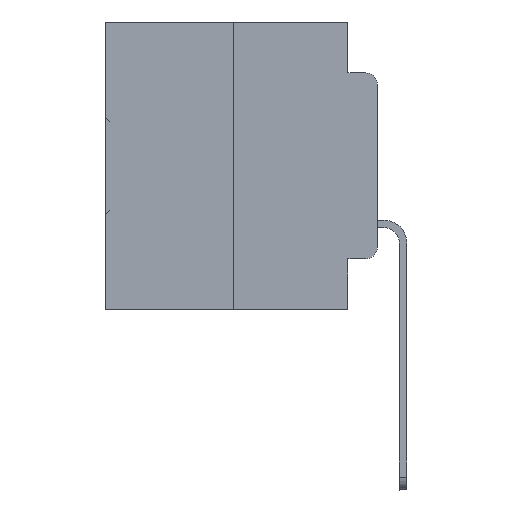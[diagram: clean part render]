
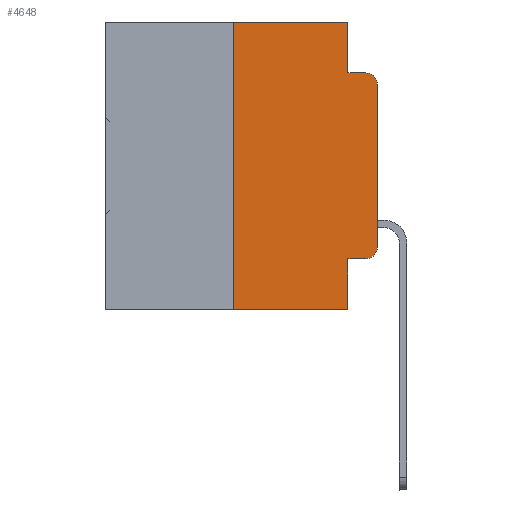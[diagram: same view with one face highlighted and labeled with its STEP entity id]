
A CAD part, left-side view. The second image highlights one B-rep face of the part: STEP entity #4648.
In plain terms, the highlighted planar face has unit normal (-1, 0, 0).
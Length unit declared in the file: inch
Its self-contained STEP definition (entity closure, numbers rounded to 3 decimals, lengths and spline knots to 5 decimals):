
#615 = DIRECTION ( 'NONE',  ( 0., 0., 1. ) ) ;
#1331 = CARTESIAN_POINT ( 'NONE',  ( 0., 0.051, 0. ) ) ;
#1469 = ORIENTED_EDGE ( 'NONE', *, *, #10704, .T. ) ;
#1869 = VECTOR ( 'NONE', #31342, 39.37008 ) ;
#2814 = DIRECTION ( 'NONE',  ( 0., -1., 0. ) ) ;
#2826 = LINE ( 'NONE', #29893, #21544 ) ;
#3425 = EDGE_CURVE ( 'NONE', #15774, #3738, #33092, .T. ) ;
#3437 = CARTESIAN_POINT ( 'NONE',  ( 0., 0.051, 0. ) ) ;
#3597 = VECTOR ( 'NONE', #5594, 39.37008 ) ;
#3738 = VERTEX_POINT ( 'NONE', #4892 ) ;
#3865 = DIRECTION ( 'NONE',  ( 0., 0., -1. ) ) ;
#4002 = DIRECTION ( 'NONE',  ( 0., -1., 0. ) ) ;
#4027 = CARTESIAN_POINT ( 'NONE',  ( 0., 0., -0.3915 ) ) ;
#4268 = ORIENTED_EDGE ( 'NONE', *, *, #32082, .T. ) ;
#4648 = ADVANCED_FACE ( 'NONE', ( #30995 ), #21522, .F. ) ;
#4735 = VECTOR ( 'NONE', #23062, 39.37008 ) ;
#4868 = LINE ( 'NONE', #16063, #3597 ) ;
#4892 = CARTESIAN_POINT ( 'NONE',  ( 0., 0., -0.1085 ) ) ;
#5521 = DIRECTION ( 'NONE',  ( 0., 0., -1. ) ) ;
#5594 = DIRECTION ( 'NONE',  ( 0., 0., -1. ) ) ;
#5624 = CARTESIAN_POINT ( 'NONE',  ( 0., 0.051, -0.5 ) ) ;
#6203 = CARTESIAN_POINT ( 'NONE',  ( 0., 0., 0. ) ) ;
#7692 = CARTESIAN_POINT ( 'NONE',  ( 0., 0.02, -0.1085 ) ) ;
#7804 = ORIENTED_EDGE ( 'NONE', *, *, #18047, .F. ) ;
#7806 = DIRECTION ( 'NONE',  ( 0., -1., 0. ) ) ;
#7923 = VERTEX_POINT ( 'NONE', #8328 ) ;
#8036 = DIRECTION ( 'NONE',  ( -1., 0., 0. ) ) ;
#8328 = CARTESIAN_POINT ( 'NONE',  ( 0., 0.051, -0.0885 ) ) ;
#8607 = VERTEX_POINT ( 'NONE', #9517 ) ;
#9348 = CARTESIAN_POINT ( 'NONE',  ( 0., 0.051, -0.4115 ) ) ;
#9517 = CARTESIAN_POINT ( 'NONE',  ( 0., 0.25, 0. ) ) ;
#10704 = EDGE_CURVE ( 'NONE', #3738, #27448, #32208, .T. ) ;
#12398 = CARTESIAN_POINT ( 'NONE',  ( 0., 0.473, 0. ) ) ;
#13071 = EDGE_CURVE ( 'NONE', #34007, #15774, #15194, .T. ) ;
#13586 = AXIS2_PLACEMENT_3D ( 'NONE', #26766, #8036, #5521 ) ;
#14562 = VECTOR ( 'NONE', #7806, 39.37008 ) ;
#14637 = ORIENTED_EDGE ( 'NONE', *, *, #22828, .F. ) ;
#15033 = VERTEX_POINT ( 'NONE', #9348 ) ;
#15194 = CIRCLE ( 'NONE', #13586, 0.02 ) ;
#15311 = CARTESIAN_POINT ( 'NONE',  ( 0., 0.051, -0.0885 ) ) ;
#15455 = CARTESIAN_POINT ( 'NONE',  ( 0., 0.02, -0.4115 ) ) ;
#15774 = VERTEX_POINT ( 'NONE', #4027 ) ;
#15840 = ORIENTED_EDGE ( 'NONE', *, *, #13071, .T. ) ;
#16063 = CARTESIAN_POINT ( 'NONE',  ( 0., 0.051, 0. ) ) ;
#16292 = LINE ( 'NONE', #34874, #14562 ) ;
#16405 = ORIENTED_EDGE ( 'NONE', *, *, #17182, .F. ) ;
#16869 = ORIENTED_EDGE ( 'NONE', *, *, #30936, .F. ) ;
#17135 = DIRECTION ( 'NONE',  ( 1., 0., 0. ) ) ;
#17182 = EDGE_CURVE ( 'NONE', #7923, #27448, #31737, .T. ) ;
#18047 = EDGE_CURVE ( 'NONE', #8607, #31022, #32504, .T. ) ;
#18884 = LINE ( 'NONE', #29030, #1869 ) ;
#20342 = EDGE_LOOP ( 'NONE', ( #35032, #1469, #16405, #14637, #7804, #20823, #22057, #16869, #4268, #15840 ) ) ;
#20721 = CARTESIAN_POINT ( 'NONE',  ( 0., 0.02, -0.0885 ) ) ;
#20823 = ORIENTED_EDGE ( 'NONE', *, *, #31244, .F. ) ;
#21342 = AXIS2_PLACEMENT_3D ( 'NONE', #7692, #29465, #24282 ) ;
#21522 = PLANE ( 'NONE',  #34302 ) ;
#21544 = VECTOR ( 'NONE', #32364, 39.37008 ) ;
#22057 = ORIENTED_EDGE ( 'NONE', *, *, #25578, .T. ) ;
#22542 = LINE ( 'NONE', #1331, #4735 ) ;
#22828 = EDGE_CURVE ( 'NONE', #31022, #7923, #22542, .T. ) ;
#22846 = CARTESIAN_POINT ( 'NONE',  ( 0., 0.473, 0. ) ) ;
#23062 = DIRECTION ( 'NONE',  ( 0., 0., -1. ) ) ;
#23066 = CARTESIAN_POINT ( 'NONE',  ( 0., 0.25, -0.5 ) ) ;
#24282 = DIRECTION ( 'NONE',  ( 0., 0., -1. ) ) ;
#24294 = VERTEX_POINT ( 'NONE', #5624 ) ;
#25578 = EDGE_CURVE ( 'NONE', #32484, #24294, #2826, .T. ) ;
#25815 = VECTOR ( 'NONE', #4002, 39.37008 ) ;
#26466 = VECTOR ( 'NONE', #615, 39.37008 ) ;
#26766 = CARTESIAN_POINT ( 'NONE',  ( 0., 0.02, -0.3915 ) ) ;
#27448 = VERTEX_POINT ( 'NONE', #20721 ) ;
#29030 = CARTESIAN_POINT ( 'NONE',  ( 0., 0.25, 0. ) ) ;
#29465 = DIRECTION ( 'NONE',  ( -1., 0., 0. ) ) ;
#29893 = CARTESIAN_POINT ( 'NONE',  ( 0., 0.473, -0.5 ) ) ;
#30035 = VECTOR ( 'NONE', #2814, 39.37008 ) ;
#30936 = EDGE_CURVE ( 'NONE', #15033, #24294, #4868, .T. ) ;
#30995 = FACE_OUTER_BOUND ( 'NONE', #20342, .T. ) ;
#31022 = VERTEX_POINT ( 'NONE', #3437 ) ;
#31244 = EDGE_CURVE ( 'NONE', #32484, #8607, #18884, .T. ) ;
#31342 = DIRECTION ( 'NONE',  ( 0., 0., 1. ) ) ;
#31737 = LINE ( 'NONE', #15311, #30035 ) ;
#32082 = EDGE_CURVE ( 'NONE', #15033, #34007, #16292, .T. ) ;
#32208 = CIRCLE ( 'NONE', #21342, 0.02 ) ;
#32364 = DIRECTION ( 'NONE',  ( 0., -1., 0. ) ) ;
#32484 = VERTEX_POINT ( 'NONE', #23066 ) ;
#32504 = LINE ( 'NONE', #12398, #25815 ) ;
#33092 = LINE ( 'NONE', #6203, #26466 ) ;
#34007 = VERTEX_POINT ( 'NONE', #15455 ) ;
#34302 = AXIS2_PLACEMENT_3D ( 'NONE', #22846, #17135, #3865 ) ;
#34874 = CARTESIAN_POINT ( 'NONE',  ( 0., 0.051, -0.4115 ) ) ;
#35032 = ORIENTED_EDGE ( 'NONE', *, *, #3425, .T. ) ;
